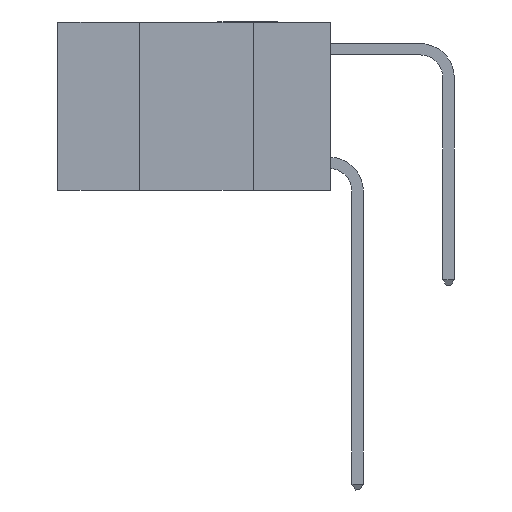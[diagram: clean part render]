
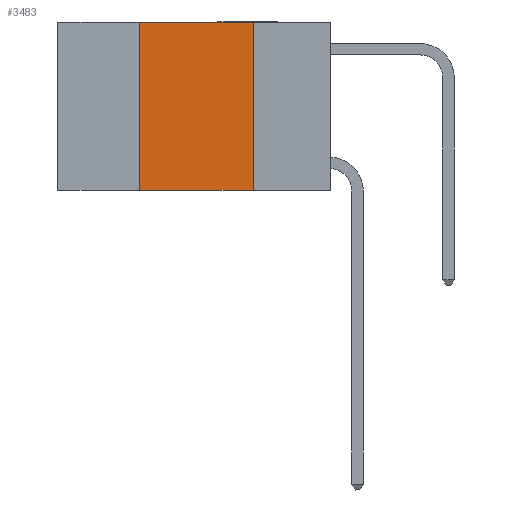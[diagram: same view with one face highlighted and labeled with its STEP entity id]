
A CAD part, left-side view. The second image highlights one B-rep face of the part: STEP entity #3483.
In plain terms, the highlighted planar face has unit normal (-1, 0, 0).
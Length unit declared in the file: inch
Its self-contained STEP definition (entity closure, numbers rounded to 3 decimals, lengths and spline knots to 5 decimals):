
#755 = DIRECTION ( 'NONE',  ( 1., 0., 0. ) ) ;
#854 = VECTOR ( 'NONE', #5483, 39.37008 ) ;
#1005 = VECTOR ( 'NONE', #3116, 39.37008 ) ;
#1015 = LINE ( 'NONE', #10361, #10358 ) ;
#1115 = CARTESIAN_POINT ( 'NONE',  ( 0., 0.17, -0.37 ) ) ;
#1389 = LINE ( 'NONE', #10742, #6219 ) ;
#1790 = CARTESIAN_POINT ( 'NONE',  ( 0., 0.42, -0.37 ) ) ;
#2500 = EDGE_CURVE ( 'NONE', #10918, #6124, #1389, .T. ) ;
#2701 = ORIENTED_EDGE ( 'NONE', *, *, #8759, .F. ) ;
#2839 = ORIENTED_EDGE ( 'NONE', *, *, #9015, .F. ) ;
#2871 = ORIENTED_EDGE ( 'NONE', *, *, #8536, .F. ) ;
#3013 = ORIENTED_EDGE ( 'NONE', *, *, #2500, .T. ) ;
#3116 = DIRECTION ( 'NONE',  ( 0., -1., 0. ) ) ;
#3248 = CARTESIAN_POINT ( 'NONE',  ( 0., 0.42, 0. ) ) ;
#3426 = PLANE ( 'NONE',  #9615 ) ;
#3448 = VERTEX_POINT ( 'NONE', #6128 ) ;
#3483 = ADVANCED_FACE ( 'NONE', ( #11645 ), #3426, .F. ) ;
#3615 = EDGE_LOOP ( 'NONE', ( #2701, #2839, #2871, #3013 ) ) ;
#3651 = CARTESIAN_POINT ( 'NONE',  ( 0., 0.17, 0. ) ) ;
#4103 = DIRECTION ( 'NONE',  ( 0., 0., 1. ) ) ;
#5378 = DIRECTION ( 'NONE',  ( 0., -1., 0. ) ) ;
#5483 = DIRECTION ( 'NONE',  ( 0., 0., -1. ) ) ;
#5696 = LINE ( 'NONE', #3651, #854 ) ;
#6124 = VERTEX_POINT ( 'NONE', #1115 ) ;
#6128 = CARTESIAN_POINT ( 'NONE',  ( 0., 0.17, 0. ) ) ;
#6200 = CARTESIAN_POINT ( 'NONE',  ( 0., 0.6, 0. ) ) ;
#6219 = VECTOR ( 'NONE', #5378, 39.37008 ) ;
#6378 = VERTEX_POINT ( 'NONE', #3248 ) ;
#7157 = DIRECTION ( 'NONE',  ( 0., 0., -1. ) ) ;
#7988 = LINE ( 'NONE', #8565, #1005 ) ;
#8536 = EDGE_CURVE ( 'NONE', #10918, #6378, #1015, .T. ) ;
#8565 = CARTESIAN_POINT ( 'NONE',  ( 0., 0.6, 0. ) ) ;
#8759 = EDGE_CURVE ( 'NONE', #3448, #6124, #5696, .T. ) ;
#9015 = EDGE_CURVE ( 'NONE', #6378, #3448, #7988, .T. ) ;
#9615 = AXIS2_PLACEMENT_3D ( 'NONE', #6200, #755, #7157 ) ;
#10358 = VECTOR ( 'NONE', #4103, 39.37008 ) ;
#10361 = CARTESIAN_POINT ( 'NONE',  ( 0., 0.42, 0. ) ) ;
#10742 = CARTESIAN_POINT ( 'NONE',  ( 0., 0.6, -0.37 ) ) ;
#10918 = VERTEX_POINT ( 'NONE', #1790 ) ;
#11645 = FACE_OUTER_BOUND ( 'NONE', #3615, .T. ) ;
